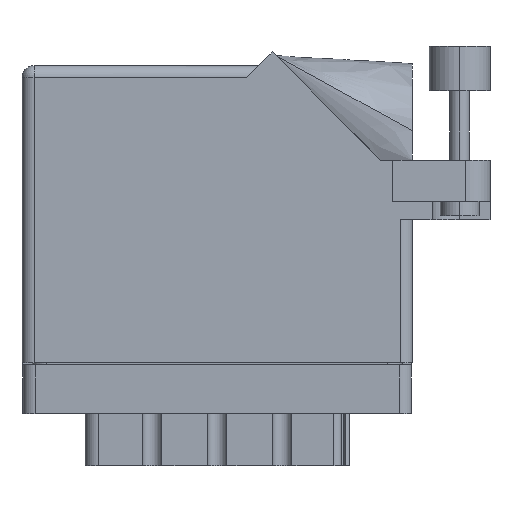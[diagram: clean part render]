
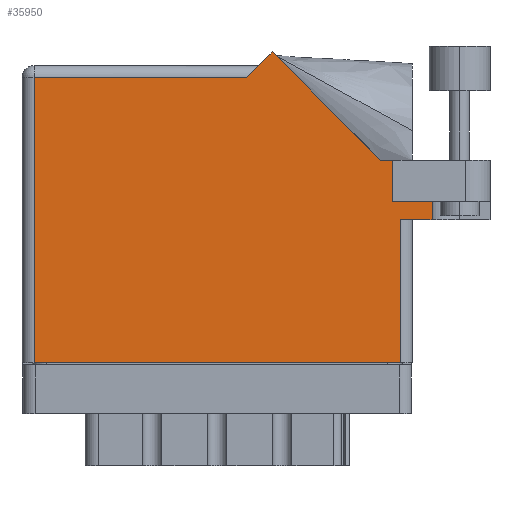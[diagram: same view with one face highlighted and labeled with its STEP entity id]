
A CAD part, front view. The second image highlights one B-rep face of the part: STEP entity #35950.
In plain terms, the highlighted face is planar.
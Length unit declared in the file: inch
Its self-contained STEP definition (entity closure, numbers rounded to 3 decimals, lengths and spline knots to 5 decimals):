
#64 = ORIENTED_EDGE ( 'NONE', *, *, #17234, .T. ) ;
#348 = CARTESIAN_POINT ( 'NONE',  ( 1.91, 0.831, 0. ) ) ;
#376 = VECTOR ( 'NONE', #25136, 39.37008 ) ;
#600 = CARTESIAN_POINT ( 'NONE',  ( 0., 0., 0. ) ) ;
#1659 = FACE_OUTER_BOUND ( 'NONE', #18304, .T. ) ;
#1956 = CARTESIAN_POINT ( 'NONE',  ( 0.062, 0., 0. ) ) ;
#2084 = DIRECTION ( 'NONE',  ( 0., -1., 0. ) ) ;
#2201 = LINE ( 'NONE', #348, #18021 ) ;
#2492 = ORIENTED_EDGE ( 'NONE', *, *, #34694, .F. ) ;
#3633 = LINE ( 'NONE', #37192, #25822 ) ;
#3689 = EDGE_CURVE ( 'NONE', #7351, #9584, #20755, .T. ) ;
#3858 = LINE ( 'NONE', #5566, #14675 ) ;
#3881 = CARTESIAN_POINT ( 'NONE',  ( 1.948, 0., 0. ) ) ;
#4281 = EDGE_CURVE ( 'NONE', #15455, #16375, #13466, .T. ) ;
#4456 = DIRECTION ( 'NONE',  ( -0.707, -0.707, 0. ) ) ;
#4997 = DIRECTION ( 'NONE',  ( -1., 0., 0. ) ) ;
#5206 = CARTESIAN_POINT ( 'NONE',  ( 0.062, 0., 0. ) ) ;
#5326 = LINE ( 'NONE', #7642, #376 ) ;
#5455 = ORIENTED_EDGE ( 'NONE', *, *, #8798, .T. ) ;
#5566 = CARTESIAN_POINT ( 'NONE',  ( 1.948, 0.737, 0. ) ) ;
#5848 = VECTOR ( 'NONE', #35676, 39.37008 ) ;
#5922 = DIRECTION ( 'NONE',  ( 0., -1., 0. ) ) ;
#6247 = VECTOR ( 'NONE', #26922, 39.37008 ) ;
#6280 = DIRECTION ( 'NONE',  ( -1., 0., 0. ) ) ;
#7351 = VERTEX_POINT ( 'NONE', #5206 ) ;
#7550 = CARTESIAN_POINT ( 'NONE',  ( 0., 1.53, 0. ) ) ;
#7642 = CARTESIAN_POINT ( 'NONE',  ( 1.84442, 1.044, 0. ) ) ;
#8099 = EDGE_CURVE ( 'NONE', #21182, #21964, #3633, .T. ) ;
#8105 = VECTOR ( 'NONE', #32295, 39.37008 ) ;
#8563 = LINE ( 'NONE', #32750, #5848 ) ;
#8798 = EDGE_CURVE ( 'NONE', #34112, #25410, #23532, .T. ) ;
#9148 = ORIENTED_EDGE ( 'NONE', *, *, #4281, .T. ) ;
#9295 = CARTESIAN_POINT ( 'NONE',  ( 2.01, 0.737, 0. ) ) ;
#9501 = CARTESIAN_POINT ( 'NONE',  ( 2.1115, 0.737, 0. ) ) ;
#9584 = VERTEX_POINT ( 'NONE', #3881 ) ;
#9831 = VERTEX_POINT ( 'NONE', #31101 ) ;
#10484 = ORIENTED_EDGE ( 'NONE', *, *, #26024, .T. ) ;
#10605 = ORIENTED_EDGE ( 'NONE', *, *, #27486, .T. ) ;
#10677 = PLANE ( 'NONE',  #28100 ) ;
#13067 = VERTEX_POINT ( 'NONE', #17758 ) ;
#13466 = LINE ( 'NONE', #30557, #24350 ) ;
#13977 = EDGE_CURVE ( 'NONE', #16375, #13067, #8563, .T. ) ;
#14675 = VECTOR ( 'NONE', #19501, 39.37008 ) ;
#15455 = VERTEX_POINT ( 'NONE', #20909 ) ;
#16375 = VERTEX_POINT ( 'NONE', #17460 ) ;
#17234 = EDGE_CURVE ( 'NONE', #25410, #9831, #37321, .T. ) ;
#17460 = CARTESIAN_POINT ( 'NONE',  ( 1.155, 1.468, 0. ) ) ;
#17758 = CARTESIAN_POINT ( 'NONE',  ( 0.062, 1.468, 0. ) ) ;
#17930 = ORIENTED_EDGE ( 'NONE', *, *, #25823, .T. ) ;
#17982 = VERTEX_POINT ( 'NONE', #18599 ) ;
#18021 = VECTOR ( 'NONE', #20572, 39.37008 ) ;
#18304 = EDGE_LOOP ( 'NONE', ( #26749, #10605, #17930, #34382, #2492, #5455, #64, #10484, #9148, #29497, #21660 ) ) ;
#18599 = CARTESIAN_POINT ( 'NONE',  ( 1.948, 0.737, 0. ) ) ;
#19501 = DIRECTION ( 'NONE',  ( 0., 1., 0. ) ) ;
#20572 = DIRECTION ( 'NONE',  ( 1., 0., 0. ) ) ;
#20755 = LINE ( 'NONE', #600, #37506 ) ;
#20909 = CARTESIAN_POINT ( 'NONE',  ( 1.28771, 1.60071, 0. ) ) ;
#21182 = VERTEX_POINT ( 'NONE', #37293 ) ;
#21660 = ORIENTED_EDGE ( 'NONE', *, *, #26055, .T. ) ;
#21964 = VERTEX_POINT ( 'NONE', #9501 ) ;
#23532 = LINE ( 'NONE', #26355, #8105 ) ;
#23628 = CARTESIAN_POINT ( 'NONE',  ( 2.41, 1.044, 0. ) ) ;
#24350 = VECTOR ( 'NONE', #4456, 39.37008 ) ;
#25136 = DIRECTION ( 'NONE',  ( -0.707, 0.707, 0. ) ) ;
#25410 = VERTEX_POINT ( 'NONE', #27190 ) ;
#25725 = VECTOR ( 'NONE', #2084, 39.37008 ) ;
#25822 = VECTOR ( 'NONE', #5922, 39.37008 ) ;
#25823 = EDGE_CURVE ( 'NONE', #17982, #21964, #36625, .T. ) ;
#26024 = EDGE_CURVE ( 'NONE', #9831, #15455, #5326, .T. ) ;
#26055 = EDGE_CURVE ( 'NONE', #13067, #7351, #33425, .T. ) ;
#26355 = CARTESIAN_POINT ( 'NONE',  ( 1.91, 0.831, 0. ) ) ;
#26484 = VECTOR ( 'NONE', #6280, 39.37008 ) ;
#26749 = ORIENTED_EDGE ( 'NONE', *, *, #3689, .T. ) ;
#26922 = DIRECTION ( 'NONE',  ( 1., 0., 0. ) ) ;
#27172 = DIRECTION ( 'NONE',  ( 1., 0., 0. ) ) ;
#27190 = CARTESIAN_POINT ( 'NONE',  ( 1.91, 1.044, 0. ) ) ;
#27486 = EDGE_CURVE ( 'NONE', #9584, #17982, #3858, .T. ) ;
#28100 = AXIS2_PLACEMENT_3D ( 'NONE', #7550, #33871, #4997 ) ;
#29497 = ORIENTED_EDGE ( 'NONE', *, *, #13977, .T. ) ;
#30557 = CARTESIAN_POINT ( 'NONE',  ( 1.217, 1.53, 0. ) ) ;
#31101 = CARTESIAN_POINT ( 'NONE',  ( 1.84442, 1.044, 0. ) ) ;
#32295 = DIRECTION ( 'NONE',  ( 0., 1., 0. ) ) ;
#32750 = CARTESIAN_POINT ( 'NONE',  ( 0., 1.468, 0. ) ) ;
#33425 = LINE ( 'NONE', #1956, #25725 ) ;
#33871 = DIRECTION ( 'NONE',  ( 0., 0., -1. ) ) ;
#34040 = CARTESIAN_POINT ( 'NONE',  ( 1.91, 0.831, 0. ) ) ;
#34112 = VERTEX_POINT ( 'NONE', #34040 ) ;
#34382 = ORIENTED_EDGE ( 'NONE', *, *, #8099, .F. ) ;
#34694 = EDGE_CURVE ( 'NONE', #34112, #21182, #2201, .T. ) ;
#35676 = DIRECTION ( 'NONE',  ( -1., 0., 0. ) ) ;
#35950 = ADVANCED_FACE ( 'NONE', ( #1659 ), #10677, .F. ) ;
#36625 = LINE ( 'NONE', #9295, #6247 ) ;
#37192 = CARTESIAN_POINT ( 'NONE',  ( 2.1115, 1.16177, 0. ) ) ;
#37293 = CARTESIAN_POINT ( 'NONE',  ( 2.1115, 0.831, 0. ) ) ;
#37321 = LINE ( 'NONE', #23628, #26484 ) ;
#37506 = VECTOR ( 'NONE', #27172, 39.37008 ) ;
